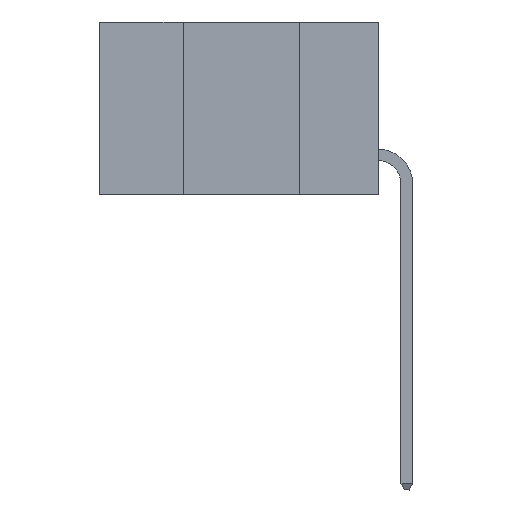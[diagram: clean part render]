
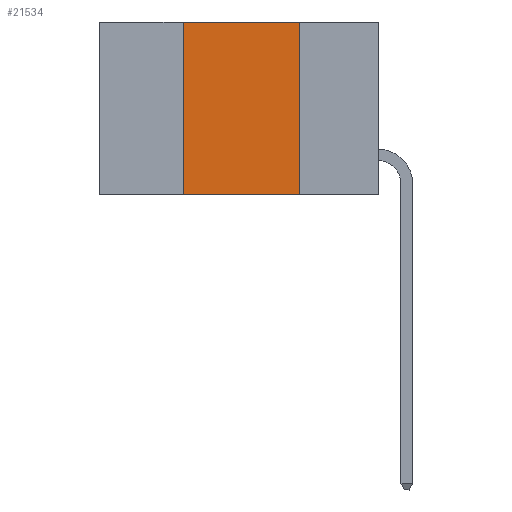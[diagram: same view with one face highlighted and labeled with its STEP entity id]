
A CAD part, left-side view. The second image highlights one B-rep face of the part: STEP entity #21534.
In plain terms, the highlighted planar face has unit normal (-1, 0, 0).
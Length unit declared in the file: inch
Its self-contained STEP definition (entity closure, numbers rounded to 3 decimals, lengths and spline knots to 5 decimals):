
#1778 = DIRECTION ( 'NONE',  ( 0., 0., 1. ) ) ;
#2311 = VERTEX_POINT ( 'NONE', #4366 ) ;
#3365 = CARTESIAN_POINT ( 'NONE',  ( 0., 0.6, -0.37 ) ) ;
#3978 = CARTESIAN_POINT ( 'NONE',  ( 0., 0.42, -0.37 ) ) ;
#4366 = CARTESIAN_POINT ( 'NONE',  ( 0., 0.17, 0. ) ) ;
#5131 = VERTEX_POINT ( 'NONE', #14294 ) ;
#5145 = DIRECTION ( 'NONE',  ( 0., 0., -1. ) ) ;
#6496 = AXIS2_PLACEMENT_3D ( 'NONE', #15460, #15588, #21457 ) ;
#6567 = DIRECTION ( 'NONE',  ( 0., -1., 0. ) ) ;
#7473 = LINE ( 'NONE', #3365, #19967 ) ;
#7667 = VERTEX_POINT ( 'NONE', #13131 ) ;
#8070 = VECTOR ( 'NONE', #1778, 39.37008 ) ;
#8994 = LINE ( 'NONE', #24817, #12470 ) ;
#9720 = VECTOR ( 'NONE', #6567, 39.37008 ) ;
#10095 = VERTEX_POINT ( 'NONE', #3978 ) ;
#11089 = ORIENTED_EDGE ( 'NONE', *, *, #24567, .F. ) ;
#11422 = ORIENTED_EDGE ( 'NONE', *, *, #15970, .F. ) ;
#12470 = VECTOR ( 'NONE', #5145, 39.37008 ) ;
#12896 = CARTESIAN_POINT ( 'NONE',  ( 0., 0.6, 0. ) ) ;
#13028 = ORIENTED_EDGE ( 'NONE', *, *, #22340, .T. ) ;
#13131 = CARTESIAN_POINT ( 'NONE',  ( 0., 0.42, 0. ) ) ;
#13261 = DIRECTION ( 'NONE',  ( 0., -1., 0. ) ) ;
#14294 = CARTESIAN_POINT ( 'NONE',  ( 0., 0.17, -0.37 ) ) ;
#15460 = CARTESIAN_POINT ( 'NONE',  ( 0., 0.6, 0. ) ) ;
#15588 = DIRECTION ( 'NONE',  ( 1., 0., 0. ) ) ;
#15970 = EDGE_CURVE ( 'NONE', #7667, #2311, #16974, .T. ) ;
#16613 = EDGE_CURVE ( 'NONE', #10095, #7667, #20020, .T. ) ;
#16974 = LINE ( 'NONE', #12896, #9720 ) ;
#17414 = ORIENTED_EDGE ( 'NONE', *, *, #16613, .F. ) ;
#17553 = FACE_OUTER_BOUND ( 'NONE', #23703, .T. ) ;
#18201 = CARTESIAN_POINT ( 'NONE',  ( 0., 0.42, -0.37 ) ) ;
#19967 = VECTOR ( 'NONE', #13261, 39.37008 ) ;
#20020 = LINE ( 'NONE', #18201, #8070 ) ;
#21457 = DIRECTION ( 'NONE',  ( 0., 0., -1. ) ) ;
#21534 = ADVANCED_FACE ( 'NONE', ( #17553 ), #25374, .F. ) ;
#22340 = EDGE_CURVE ( 'NONE', #10095, #5131, #7473, .T. ) ;
#23703 = EDGE_LOOP ( 'NONE', ( #11089, #11422, #17414, #13028 ) ) ;
#24567 = EDGE_CURVE ( 'NONE', #2311, #5131, #8994, .T. ) ;
#24817 = CARTESIAN_POINT ( 'NONE',  ( 0., 0.17, -0.37 ) ) ;
#25374 = PLANE ( 'NONE',  #6496 ) ;
